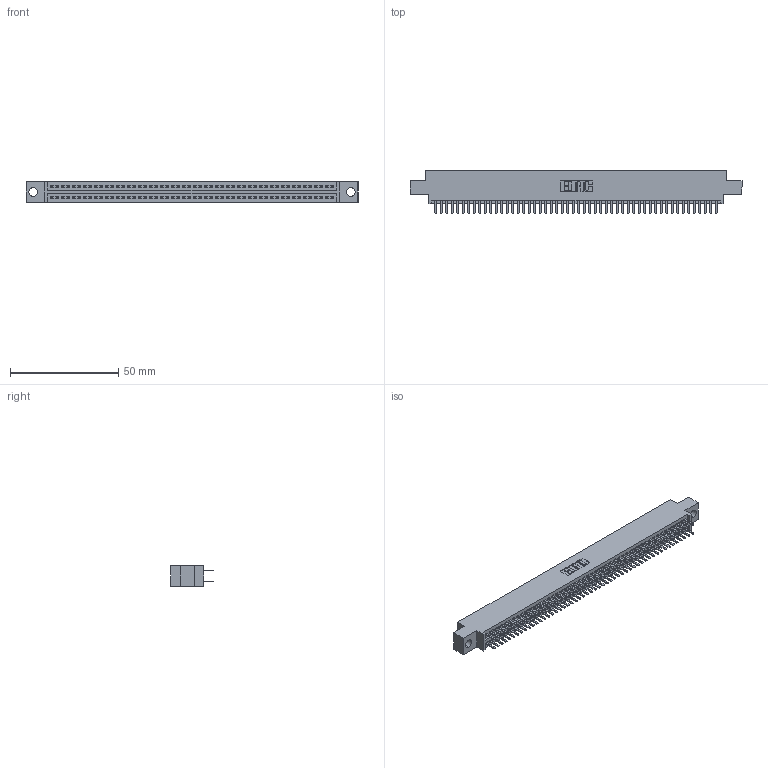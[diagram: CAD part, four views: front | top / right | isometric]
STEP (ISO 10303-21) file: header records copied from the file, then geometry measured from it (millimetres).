
FILE_DESCRIPTION (( 'STEP AP203' ), '1' );
FILE_NAME ('395-104-520-804.STEP', '2021-06-17T15:53:55', ( '' ), ( '' ), 'SwSTEP 2.0', 'SolidWorks 2020', '' );
FILE_SCHEMA (( 'CONFIG_CONTROL_DESIGN' ));
Length unit declared in the file: inch
Products named in the file (3): 345 Part_0.170 Offset - 0.156 Dia-TI; 345-292-001_345-293-120; 395-104-520-804
Assembly tree (105 placements, depth 2):
  395-104-520-804
    345 Part_0.170 Offset - 0.156 Dia-TI
    345-292-001_345-293-120  x104
Bounding box: 153.29 x 19.68 x 9.4 mm (x, y, z)
Volume: 14718.4 mm3; surface area: 21847.8 mm2
Topology: 105 solids, 105 shells, 5760 faces, 16717 edges, 10866 vertices
Faces by surface type: plane 3738, cylinder 2022
Entity records: 40119 total; most frequent: CARTESIAN_POINT 6734, ORIENTED_EDGE 6654, DIRECTION 5911, EDGE_CURVE 3327, VECTOR 2983, LINE 2983, VERTEX_POINT 2214, AXIS2_PLACEMENT_3D 1464
